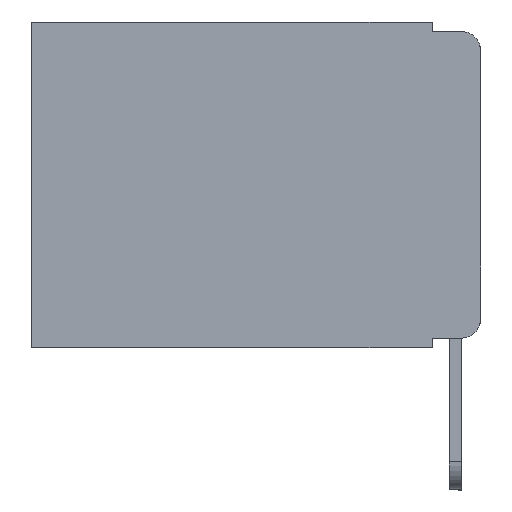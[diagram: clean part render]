
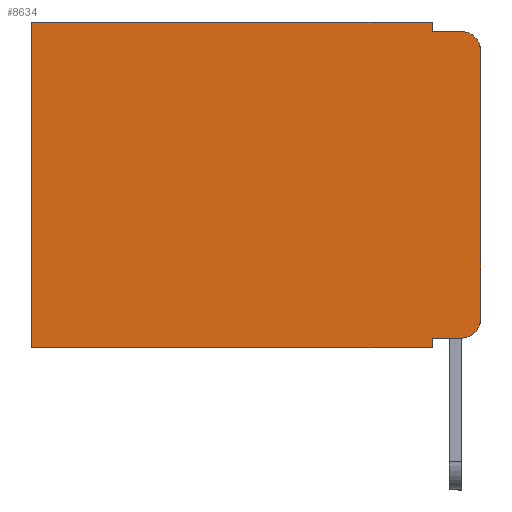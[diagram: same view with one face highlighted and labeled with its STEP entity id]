
A CAD part, left-side view. The second image highlights one B-rep face of the part: STEP entity #8634.
In plain terms, the highlighted planar face has unit normal (-1, 0, 0).
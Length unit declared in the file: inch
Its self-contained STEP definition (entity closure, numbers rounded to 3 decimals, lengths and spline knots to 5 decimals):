
#636 = CARTESIAN_POINT ( 'NONE',  ( 0.298, 0., -0.343 ) ) ;
#644 = ORIENTED_EDGE ( 'NONE', *, *, #11305, .T. ) ;
#776 = DIRECTION ( 'NONE',  ( 0., 1., 0. ) ) ;
#1284 = EDGE_CURVE ( 'NONE', #15963, #6337, #6266, .T. ) ;
#1408 = ORIENTED_EDGE ( 'NONE', *, *, #9959, .T. ) ;
#1881 = AXIS2_PLACEMENT_3D ( 'NONE', #12980, #14485, #11464 ) ;
#1898 = DIRECTION ( 'NONE',  ( 0., 0., -1. ) ) ;
#2406 = CARTESIAN_POINT ( 'NONE',  ( 0.298, 0.051, 0. ) ) ;
#2433 = DIRECTION ( 'NONE',  ( 0., 0., -1. ) ) ;
#2822 = LINE ( 'NONE', #7123, #16378 ) ;
#3415 = CARTESIAN_POINT ( 'NONE',  ( 0.298, 0.473, -0.343 ) ) ;
#3622 = LINE ( 'NONE', #6304, #7308 ) ;
#3625 = LINE ( 'NONE', #6808, #14844 ) ;
#3916 = DIRECTION ( 'NONE',  ( 0., -1., 0. ) ) ;
#3978 = VERTEX_POINT ( 'NONE', #13272 ) ;
#4077 = ORIENTED_EDGE ( 'NONE', *, *, #1284, .T. ) ;
#4127 = DIRECTION ( 'NONE',  ( 0., -1., 0. ) ) ;
#4231 = CARTESIAN_POINT ( 'NONE',  ( 0.298, 0., 0. ) ) ;
#4321 = EDGE_CURVE ( 'NONE', #15963, #9873, #18633, .T. ) ;
#4648 = VECTOR ( 'NONE', #12755, 39.37008 ) ;
#4764 = EDGE_LOOP ( 'NONE', ( #13181, #4077, #15016, #8437, #644, #18420, #8417, #16754, #1408, #7458 ) ) ;
#4791 = EDGE_CURVE ( 'NONE', #9751, #16923, #8742, .T. ) ;
#4892 = CARTESIAN_POINT ( 'NONE',  ( 0.298, 0., 0. ) ) ;
#5349 = LINE ( 'NONE', #19197, #11160 ) ;
#5623 = PLANE ( 'NONE',  #11862 ) ;
#5719 = CARTESIAN_POINT ( 'NONE',  ( 0.298, 0., 0. ) ) ;
#5857 = VERTEX_POINT ( 'NONE', #6179 ) ;
#6041 = EDGE_CURVE ( 'NONE', #18214, #15882, #5349, .T. ) ;
#6106 = EDGE_CURVE ( 'NONE', #11728, #9873, #8580, .T. ) ;
#6179 = CARTESIAN_POINT ( 'NONE',  ( 0.298, 0.051, -0.343 ) ) ;
#6266 = CIRCLE ( 'NONE', #12363, 0.02 ) ;
#6304 = CARTESIAN_POINT ( 'NONE',  ( 0.298, 0.051, 0. ) ) ;
#6312 = VECTOR ( 'NONE', #11751, 39.37008 ) ;
#6337 = VERTEX_POINT ( 'NONE', #11146 ) ;
#6808 = CARTESIAN_POINT ( 'NONE',  ( 0.298, 0.051, -0.01 ) ) ;
#7123 = CARTESIAN_POINT ( 'NONE',  ( 0.298, 0.051, -0.333 ) ) ;
#7308 = VECTOR ( 'NONE', #14040, 39.37008 ) ;
#7458 = ORIENTED_EDGE ( 'NONE', *, *, #6106, .T. ) ;
#8034 = EDGE_CURVE ( 'NONE', #3978, #5857, #3622, .T. ) ;
#8243 = DIRECTION ( 'NONE',  ( 0., 0., -1. ) ) ;
#8417 = ORIENTED_EDGE ( 'NONE', *, *, #15027, .F. ) ;
#8437 = ORIENTED_EDGE ( 'NONE', *, *, #6041, .F. ) ;
#8580 = CIRCLE ( 'NONE', #1881, 0.02 ) ;
#8634 = ADVANCED_FACE ( 'NONE', ( #11739 ), #5623, .F. ) ;
#8638 = DIRECTION ( 'NONE',  ( 0., 0., -1. ) ) ;
#8742 = LINE ( 'NONE', #14481, #6312 ) ;
#9485 = CARTESIAN_POINT ( 'NONE',  ( 0.298, 0., -0.03 ) ) ;
#9651 = LINE ( 'NONE', #636, #4648 ) ;
#9751 = VERTEX_POINT ( 'NONE', #14370 ) ;
#9873 = VERTEX_POINT ( 'NONE', #19375 ) ;
#9959 = EDGE_CURVE ( 'NONE', #3978, #11728, #2822, .T. ) ;
#11146 = CARTESIAN_POINT ( 'NONE',  ( 0.298, 0.02, -0.01 ) ) ;
#11159 = CARTESIAN_POINT ( 'NONE',  ( 0.298, 0.02, -0.03 ) ) ;
#11160 = VECTOR ( 'NONE', #8638, 39.37008 ) ;
#11305 = EDGE_CURVE ( 'NONE', #18214, #9751, #16641, .T. ) ;
#11464 = DIRECTION ( 'NONE',  ( 0., 0., -1. ) ) ;
#11728 = VERTEX_POINT ( 'NONE', #14647 ) ;
#11739 = FACE_OUTER_BOUND ( 'NONE', #4764, .T. ) ;
#11751 = DIRECTION ( 'NONE',  ( 0., 0., -1. ) ) ;
#11835 = DIRECTION ( 'NONE',  ( 1., 0., 0. ) ) ;
#11862 = AXIS2_PLACEMENT_3D ( 'NONE', #5719, #11835, #2433 ) ;
#12363 = AXIS2_PLACEMENT_3D ( 'NONE', #11159, #17268, #8243 ) ;
#12755 = DIRECTION ( 'NONE',  ( 0., 1., 0. ) ) ;
#12980 = CARTESIAN_POINT ( 'NONE',  ( 0.298, 0.02, -0.313 ) ) ;
#13181 = ORIENTED_EDGE ( 'NONE', *, *, #4321, .F. ) ;
#13272 = CARTESIAN_POINT ( 'NONE',  ( 0.298, 0.051, -0.333 ) ) ;
#13673 = EDGE_CURVE ( 'NONE', #15882, #6337, #3625, .T. ) ;
#14040 = DIRECTION ( 'NONE',  ( 0., 0., -1. ) ) ;
#14370 = CARTESIAN_POINT ( 'NONE',  ( 0.298, 0.473, 0. ) ) ;
#14430 = VECTOR ( 'NONE', #776, 39.37008 ) ;
#14481 = CARTESIAN_POINT ( 'NONE',  ( 0.298, 0.473, 0. ) ) ;
#14485 = DIRECTION ( 'NONE',  ( -1., 0., 0. ) ) ;
#14647 = CARTESIAN_POINT ( 'NONE',  ( 0.298, 0.02, -0.333 ) ) ;
#14844 = VECTOR ( 'NONE', #3916, 39.37008 ) ;
#15016 = ORIENTED_EDGE ( 'NONE', *, *, #13673, .F. ) ;
#15027 = EDGE_CURVE ( 'NONE', #5857, #16923, #9651, .T. ) ;
#15159 = VECTOR ( 'NONE', #1898, 39.37008 ) ;
#15882 = VERTEX_POINT ( 'NONE', #17489 ) ;
#15963 = VERTEX_POINT ( 'NONE', #9485 ) ;
#16378 = VECTOR ( 'NONE', #4127, 39.37008 ) ;
#16641 = LINE ( 'NONE', #4231, #14430 ) ;
#16754 = ORIENTED_EDGE ( 'NONE', *, *, #8034, .F. ) ;
#16923 = VERTEX_POINT ( 'NONE', #3415 ) ;
#17268 = DIRECTION ( 'NONE',  ( -1., 0., 0. ) ) ;
#17489 = CARTESIAN_POINT ( 'NONE',  ( 0.298, 0.051, -0.01 ) ) ;
#18214 = VERTEX_POINT ( 'NONE', #2406 ) ;
#18420 = ORIENTED_EDGE ( 'NONE', *, *, #4791, .T. ) ;
#18633 = LINE ( 'NONE', #4892, #15159 ) ;
#19197 = CARTESIAN_POINT ( 'NONE',  ( 0.298, 0.051, 0. ) ) ;
#19375 = CARTESIAN_POINT ( 'NONE',  ( 0.298, 0., -0.313 ) ) ;
